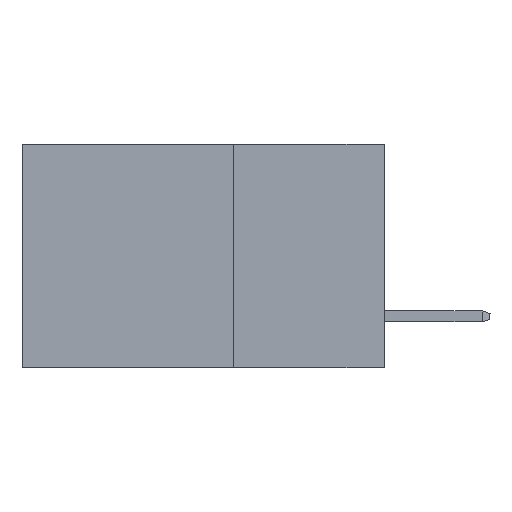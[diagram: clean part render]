
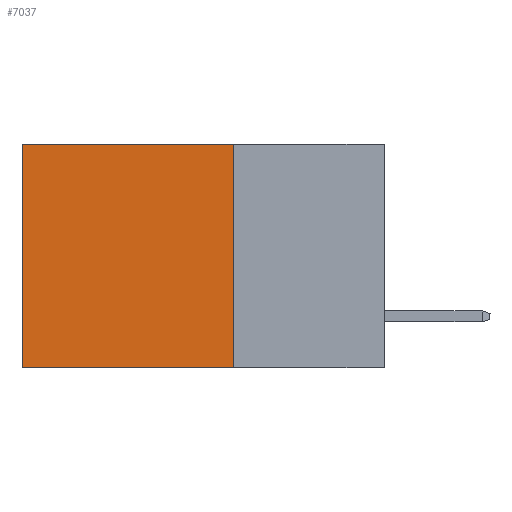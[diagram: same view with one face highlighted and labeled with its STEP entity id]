
A CAD part, left-side view. The second image highlights one B-rep face of the part: STEP entity #7037.
In plain terms, the highlighted planar face has unit normal (-1, 0, 0).
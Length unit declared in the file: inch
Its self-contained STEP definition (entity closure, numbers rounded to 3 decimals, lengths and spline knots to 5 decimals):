
#435 = VECTOR ( 'NONE', #10558, 39.37008 ) ;
#998 = EDGE_CURVE ( 'NONE', #1240, #5044, #4826, .T. ) ;
#1176 = FACE_OUTER_BOUND ( 'NONE', #2618, .T. ) ;
#1209 = EDGE_CURVE ( 'NONE', #6655, #1240, #8479, .T. ) ;
#1240 = VERTEX_POINT ( 'NONE', #10245 ) ;
#1544 = LINE ( 'NONE', #9297, #10666 ) ;
#1810 = AXIS2_PLACEMENT_3D ( 'NONE', #10613, #2783, #6281 ) ;
#2618 = EDGE_LOOP ( 'NONE', ( #3249, #5802, #6122, #7637 ) ) ;
#2783 = DIRECTION ( 'NONE',  ( 1., 0., 0. ) ) ;
#2917 = CARTESIAN_POINT ( 'NONE',  ( 0.2615, 0.6, -0.37 ) ) ;
#3123 = CARTESIAN_POINT ( 'NONE',  ( 0.2615, 0.6, -0.37 ) ) ;
#3249 = ORIENTED_EDGE ( 'NONE', *, *, #998, .T. ) ;
#3250 = VERTEX_POINT ( 'NONE', #8971 ) ;
#3701 = PLANE ( 'NONE',  #1810 ) ;
#3813 = CARTESIAN_POINT ( 'NONE',  ( 0.2615, 0.25, -0.37 ) ) ;
#4826 = LINE ( 'NONE', #2917, #6418 ) ;
#4935 = EDGE_CURVE ( 'NONE', #3250, #5044, #7069, .T. ) ;
#5044 = VERTEX_POINT ( 'NONE', #3123 ) ;
#5054 = EDGE_CURVE ( 'NONE', #6655, #3250, #1544, .T. ) ;
#5802 = ORIENTED_EDGE ( 'NONE', *, *, #4935, .F. ) ;
#6122 = ORIENTED_EDGE ( 'NONE', *, *, #5054, .F. ) ;
#6281 = DIRECTION ( 'NONE',  ( 0., 0., -1. ) ) ;
#6418 = VECTOR ( 'NONE', #10915, 39.37008 ) ;
#6655 = VERTEX_POINT ( 'NONE', #10844 ) ;
#7037 = ADVANCED_FACE ( 'NONE', ( #1176 ), #3701, .F. ) ;
#7069 = LINE ( 'NONE', #3813, #435 ) ;
#7595 = DIRECTION ( 'NONE',  ( 0., 0., -1. ) ) ;
#7637 = ORIENTED_EDGE ( 'NONE', *, *, #1209, .T. ) ;
#8479 = LINE ( 'NONE', #11144, #10384 ) ;
#8971 = CARTESIAN_POINT ( 'NONE',  ( 0.2615, 0.25, -0.37 ) ) ;
#9297 = CARTESIAN_POINT ( 'NONE',  ( 0.2615, 0.25, -0.37 ) ) ;
#9378 = DIRECTION ( 'NONE',  ( 0., 1., 0. ) ) ;
#10245 = CARTESIAN_POINT ( 'NONE',  ( 0.2615, 0.6, 0. ) ) ;
#10384 = VECTOR ( 'NONE', #9378, 39.37008 ) ;
#10558 = DIRECTION ( 'NONE',  ( 0., 1., 0. ) ) ;
#10613 = CARTESIAN_POINT ( 'NONE',  ( 0.2615, 0.25, -0.37 ) ) ;
#10666 = VECTOR ( 'NONE', #7595, 39.37008 ) ;
#10844 = CARTESIAN_POINT ( 'NONE',  ( 0.2615, 0.25, 0. ) ) ;
#10915 = DIRECTION ( 'NONE',  ( 0., 0., -1. ) ) ;
#11144 = CARTESIAN_POINT ( 'NONE',  ( 0.2615, 0.25, 0. ) ) ;
